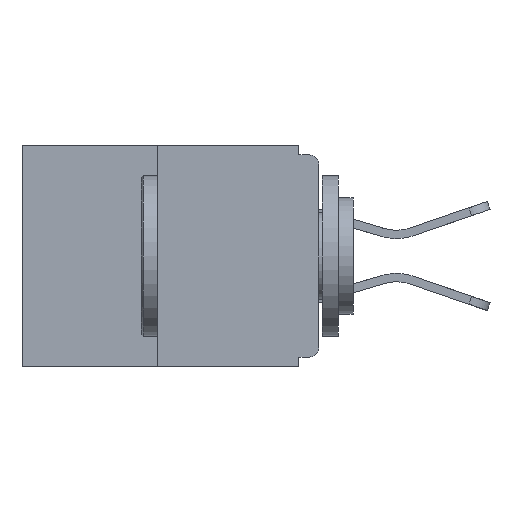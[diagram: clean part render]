
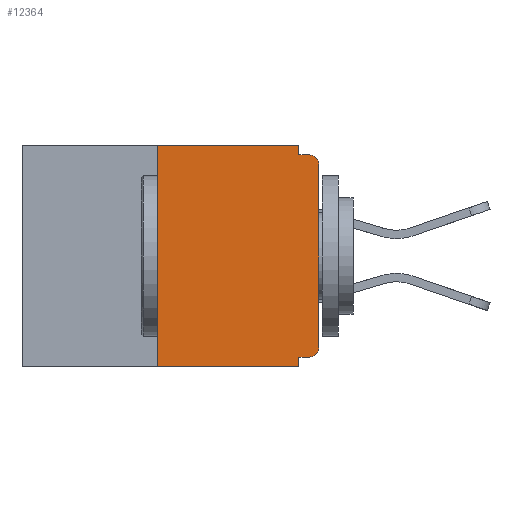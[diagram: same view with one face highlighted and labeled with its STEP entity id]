
A CAD part, left-side view. The second image highlights one B-rep face of the part: STEP entity #12364.
In plain terms, the highlighted planar face has unit normal (-1, 0, 0).
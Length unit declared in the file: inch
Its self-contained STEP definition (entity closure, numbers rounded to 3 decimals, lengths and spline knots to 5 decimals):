
#169 = LINE ( 'NONE', #907, #15617 ) ;
#472 = DIRECTION ( 'NONE',  ( 0., 0., -1. ) ) ;
#877 = FACE_OUTER_BOUND ( 'NONE', #8897, .T. ) ;
#907 = CARTESIAN_POINT ( 'NONE',  ( 0., 0.25, 0. ) ) ;
#1076 = VECTOR ( 'NONE', #5071, 39.37008 ) ;
#1286 = CARTESIAN_POINT ( 'NONE',  ( 0., 0., -0.328 ) ) ;
#1572 = ORIENTED_EDGE ( 'NONE', *, *, #13412, .F. ) ;
#1603 = CARTESIAN_POINT ( 'NONE',  ( 0., 0.25, -0.343 ) ) ;
#1675 = ORIENTED_EDGE ( 'NONE', *, *, #18817, .F. ) ;
#1712 = LINE ( 'NONE', #12857, #10076 ) ;
#1824 = ORIENTED_EDGE ( 'NONE', *, *, #12545, .F. ) ;
#1865 = VERTEX_POINT ( 'NONE', #9523 ) ;
#2007 = DIRECTION ( 'NONE',  ( -1., 0., 0. ) ) ;
#2125 = CARTESIAN_POINT ( 'NONE',  ( 0., 0.015, -0.313 ) ) ;
#2207 = ORIENTED_EDGE ( 'NONE', *, *, #7724, .T. ) ;
#2290 = CARTESIAN_POINT ( 'NONE',  ( 0., 0.46, 0. ) ) ;
#2720 = LINE ( 'NONE', #11133, #14177 ) ;
#3836 = CARTESIAN_POINT ( 'NONE',  ( 0., 0.015, -0.015 ) ) ;
#4375 = EDGE_CURVE ( 'NONE', #16693, #12437, #2720, .T. ) ;
#5041 = EDGE_CURVE ( 'NONE', #16886, #16462, #13977, .T. ) ;
#5071 = DIRECTION ( 'NONE',  ( 0., 0., -1. ) ) ;
#5103 = VERTEX_POINT ( 'NONE', #6358 ) ;
#5203 = CARTESIAN_POINT ( 'NONE',  ( 0., 0.031, 0. ) ) ;
#5243 = CARTESIAN_POINT ( 'NONE',  ( 0., 0.46, 0. ) ) ;
#5661 = AXIS2_PLACEMENT_3D ( 'NONE', #2125, #2007, #472 ) ;
#5732 = DIRECTION ( 'NONE',  ( 0., 1., 0. ) ) ;
#5933 = EDGE_CURVE ( 'NONE', #14708, #16462, #10629, .T. ) ;
#5993 = CARTESIAN_POINT ( 'NONE',  ( 0., 0.015, -0.03 ) ) ;
#6358 = CARTESIAN_POINT ( 'NONE',  ( 0., 0.25, 0. ) ) ;
#6547 = DIRECTION ( 'NONE',  ( 0., -1., 0. ) ) ;
#6941 = VECTOR ( 'NONE', #10236, 39.37008 ) ;
#7199 = VECTOR ( 'NONE', #6547, 39.37008 ) ;
#7278 = CARTESIAN_POINT ( 'NONE',  ( 0., 0.031, -0.343 ) ) ;
#7459 = CARTESIAN_POINT ( 'NONE',  ( 0., 0.031, 0. ) ) ;
#7486 = DIRECTION ( 'NONE',  ( -1., 0., 0. ) ) ;
#7680 = DIRECTION ( 'NONE',  ( 0., 0., -1. ) ) ;
#7724 = EDGE_CURVE ( 'NONE', #9394, #14708, #1712, .T. ) ;
#8542 = EDGE_CURVE ( 'NONE', #12172, #9394, #16645, .T. ) ;
#8897 = EDGE_LOOP ( 'NONE', ( #1675, #1824, #11509, #1572, #14411, #18659, #2207, #18661, #18951, #8917 ) ) ;
#8917 = ORIENTED_EDGE ( 'NONE', *, *, #13171, .F. ) ;
#9394 = VERTEX_POINT ( 'NONE', #15614 ) ;
#9520 = DIRECTION ( 'NONE',  ( 1., 0., 0. ) ) ;
#9523 = CARTESIAN_POINT ( 'NONE',  ( 0., 0.031, -0.328 ) ) ;
#9935 = LINE ( 'NONE', #5203, #1076 ) ;
#10030 = DIRECTION ( 'NONE',  ( 0., 0., 1. ) ) ;
#10076 = VECTOR ( 'NONE', #10030, 39.37008 ) ;
#10236 = DIRECTION ( 'NONE',  ( 0., 0., -1. ) ) ;
#10629 = CIRCLE ( 'NONE', #10988, 0.015 ) ;
#10988 = AXIS2_PLACEMENT_3D ( 'NONE', #5993, #7486, #7680 ) ;
#11133 = CARTESIAN_POINT ( 'NONE',  ( 0., 0.46, -0.343 ) ) ;
#11509 = ORIENTED_EDGE ( 'NONE', *, *, #4375, .T. ) ;
#12017 = LINE ( 'NONE', #2290, #15561 ) ;
#12172 = VERTEX_POINT ( 'NONE', #15985 ) ;
#12364 = ADVANCED_FACE ( 'NONE', ( #877 ), #13925, .F. ) ;
#12437 = VERTEX_POINT ( 'NONE', #13990 ) ;
#12545 = EDGE_CURVE ( 'NONE', #16693, #5103, #169, .T. ) ;
#12857 = CARTESIAN_POINT ( 'NONE',  ( 0., 0., 0. ) ) ;
#13171 = EDGE_CURVE ( 'NONE', #17360, #16886, #9935, .T. ) ;
#13412 = EDGE_CURVE ( 'NONE', #1865, #12437, #14395, .T. ) ;
#13744 = CARTESIAN_POINT ( 'NONE',  ( 0., 0., -0.03 ) ) ;
#13925 = PLANE ( 'NONE',  #16867 ) ;
#13977 = LINE ( 'NONE', #15512, #7199 ) ;
#13990 = CARTESIAN_POINT ( 'NONE',  ( 0., 0.031, -0.343 ) ) ;
#14153 = VECTOR ( 'NONE', #5732, 39.37008 ) ;
#14177 = VECTOR ( 'NONE', #15660, 39.37008 ) ;
#14315 = DIRECTION ( 'NONE',  ( 0., 0., 1. ) ) ;
#14395 = LINE ( 'NONE', #7278, #6941 ) ;
#14411 = ORIENTED_EDGE ( 'NONE', *, *, #17821, .F. ) ;
#14708 = VERTEX_POINT ( 'NONE', #13744 ) ;
#15512 = CARTESIAN_POINT ( 'NONE',  ( 0., 0., -0.015 ) ) ;
#15561 = VECTOR ( 'NONE', #15678, 39.37008 ) ;
#15614 = CARTESIAN_POINT ( 'NONE',  ( 0., 0., -0.313 ) ) ;
#15617 = VECTOR ( 'NONE', #14315, 39.37008 ) ;
#15660 = DIRECTION ( 'NONE',  ( 0., -1., 0. ) ) ;
#15678 = DIRECTION ( 'NONE',  ( 0., -1., 0. ) ) ;
#15985 = CARTESIAN_POINT ( 'NONE',  ( 0., 0.015, -0.328 ) ) ;
#16462 = VERTEX_POINT ( 'NONE', #3836 ) ;
#16645 = CIRCLE ( 'NONE', #5661, 0.015 ) ;
#16693 = VERTEX_POINT ( 'NONE', #1603 ) ;
#16867 = AXIS2_PLACEMENT_3D ( 'NONE', #5243, #9520, #18403 ) ;
#16886 = VERTEX_POINT ( 'NONE', #18480 ) ;
#17360 = VERTEX_POINT ( 'NONE', #7459 ) ;
#17821 = EDGE_CURVE ( 'NONE', #12172, #1865, #18110, .T. ) ;
#18110 = LINE ( 'NONE', #1286, #14153 ) ;
#18403 = DIRECTION ( 'NONE',  ( 0., 0., -1. ) ) ;
#18480 = CARTESIAN_POINT ( 'NONE',  ( 0., 0.031, -0.015 ) ) ;
#18659 = ORIENTED_EDGE ( 'NONE', *, *, #8542, .T. ) ;
#18661 = ORIENTED_EDGE ( 'NONE', *, *, #5933, .T. ) ;
#18817 = EDGE_CURVE ( 'NONE', #5103, #17360, #12017, .T. ) ;
#18951 = ORIENTED_EDGE ( 'NONE', *, *, #5041, .F. ) ;
